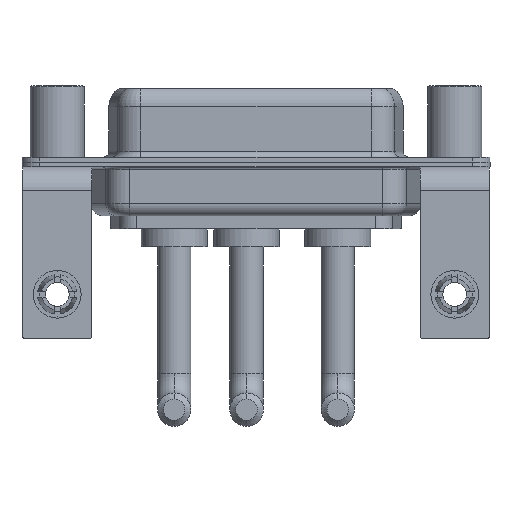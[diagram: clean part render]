
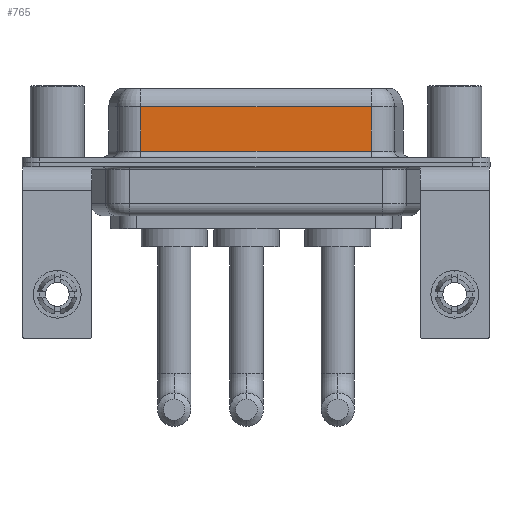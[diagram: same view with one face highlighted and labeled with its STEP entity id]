
A CAD part, front view. The second image highlights one B-rep face of the part: STEP entity #765.
In plain terms, the highlighted planar face has unit normal (0, -1, 0).
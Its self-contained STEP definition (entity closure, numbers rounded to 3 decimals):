
#765 = ADVANCED_FACE ( 'NONE', ( #17321 ), #6563, .F. ) ;
#814 = VERTEX_POINT ( 'NONE', #16113 ) ;
#870 = VERTEX_POINT ( 'NONE', #8647 ) ;
#1226 = EDGE_CURVE ( 'NONE', #1680, #870, #14697, .T. ) ;
#1240 = CARTESIAN_POINT ( 'NONE',  ( 26.287, -3.95, 4.65 ) ) ;
#1680 = VERTEX_POINT ( 'NONE', #1240 ) ;
#1841 = DIRECTION ( 'NONE',  ( 1., 0., 0. ) ) ;
#2356 = DIRECTION ( 'NONE',  ( -1., 0., 0. ) ) ;
#3930 = CARTESIAN_POINT ( 'NONE',  ( 7.013, -3.95, 6.4 ) ) ;
#4047 = AXIS2_PLACEMENT_3D ( 'NONE', #8127, #17247, #9622 ) ;
#4088 = VECTOR ( 'NONE', #12065, 1000. ) ;
#4379 = CARTESIAN_POINT ( 'NONE',  ( 26.287, -3.95, 0.9 ) ) ;
#4454 = EDGE_LOOP ( 'NONE', ( #16178, #4653, #16108, #5738 ) ) ;
#4653 = ORIENTED_EDGE ( 'NONE', *, *, #9102, .T. ) ;
#5271 = DIRECTION ( 'NONE',  ( 0., 0., -1. ) ) ;
#5738 = ORIENTED_EDGE ( 'NONE', *, *, #13148, .T. ) ;
#6497 = LINE ( 'NONE', #3930, #12658 ) ;
#6563 = PLANE ( 'NONE',  #4047 ) ;
#7644 = CARTESIAN_POINT ( 'NONE',  ( 7.013, -3.95, 0.9 ) ) ;
#8127 = CARTESIAN_POINT ( 'NONE',  ( 26.287, -3.95, 6.4 ) ) ;
#8341 = LINE ( 'NONE', #4379, #9419 ) ;
#8647 = CARTESIAN_POINT ( 'NONE',  ( 26.287, -3.95, 0.9 ) ) ;
#8722 = EDGE_CURVE ( 'NONE', #814, #14695, #6497, .T. ) ;
#9027 = LINE ( 'NONE', #14385, #10708 ) ;
#9102 = EDGE_CURVE ( 'NONE', #1680, #814, #9027, .T. ) ;
#9419 = VECTOR ( 'NONE', #1841, 1000. ) ;
#9622 = DIRECTION ( 'NONE',  ( 0., 0., 1. ) ) ;
#10708 = VECTOR ( 'NONE', #2356, 1000. ) ;
#12065 = DIRECTION ( 'NONE',  ( 0., 0., -1. ) ) ;
#12658 = VECTOR ( 'NONE', #5271, 1000. ) ;
#13148 = EDGE_CURVE ( 'NONE', #14695, #870, #8341, .T. ) ;
#14385 = CARTESIAN_POINT ( 'NONE',  ( 26.287, -3.95, 4.65 ) ) ;
#14695 = VERTEX_POINT ( 'NONE', #7644 ) ;
#14697 = LINE ( 'NONE', #15918, #4088 ) ;
#15918 = CARTESIAN_POINT ( 'NONE',  ( 26.287, -3.95, 6.4 ) ) ;
#16108 = ORIENTED_EDGE ( 'NONE', *, *, #8722, .T. ) ;
#16113 = CARTESIAN_POINT ( 'NONE',  ( 7.013, -3.95, 4.65 ) ) ;
#16178 = ORIENTED_EDGE ( 'NONE', *, *, #1226, .F. ) ;
#17247 = DIRECTION ( 'NONE',  ( 0., 1., 0. ) ) ;
#17321 = FACE_OUTER_BOUND ( 'NONE', #4454, .T. ) ;
